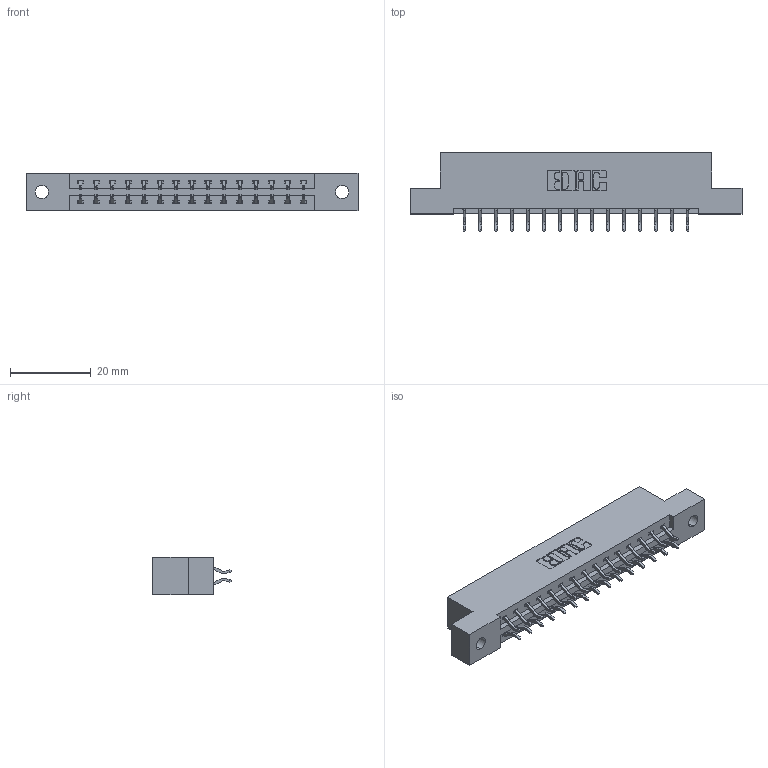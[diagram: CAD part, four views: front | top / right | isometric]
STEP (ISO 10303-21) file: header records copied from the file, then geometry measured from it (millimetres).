
FILE_DESCRIPTION (( 'STEP AP203' ), '1' );
FILE_NAME ('337-030-556-202.STEP', '2018-08-07T01:58:07', ( '' ), ( '' ), 'SwSTEP 2.0', 'SolidWorks 2016', '' );
FILE_SCHEMA (( 'CONFIG_CONTROL_DESIGN' ));
Length unit declared in the file: inch
Products named in the file (3): 337-030-556-202; 337 Part_Flush Mounting Lugs - 0.128 Dia; 345-292-001_556 Tail
Assembly tree (31 placements, depth 2):
  337-030-556-202
    337 Part_Flush Mounting Lugs - 0.128 Dia
    345-292-001_556 Tail  x30
Bounding box: 82.45 x 19.57 x 9.4 mm (x, y, z)
Volume: 8291.8 mm3; surface area: 8807.3 mm2
Topology: 31 solids, 31 shells, 1914 faces, 5681 edges, 3746 vertices
Faces by surface type: plane 1330, cylinder 584
Entity records: 15345 total; most frequent: CARTESIAN_POINT 2622, ORIENTED_EDGE 2546, DIRECTION 2269, EDGE_CURVE 1273, LINE 1137, VECTOR 1137, VERTEX_POINT 846, AXIS2_PLACEMENT_3D 566
